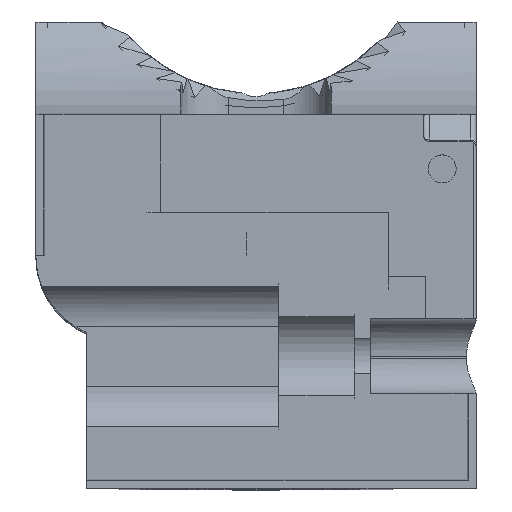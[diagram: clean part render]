
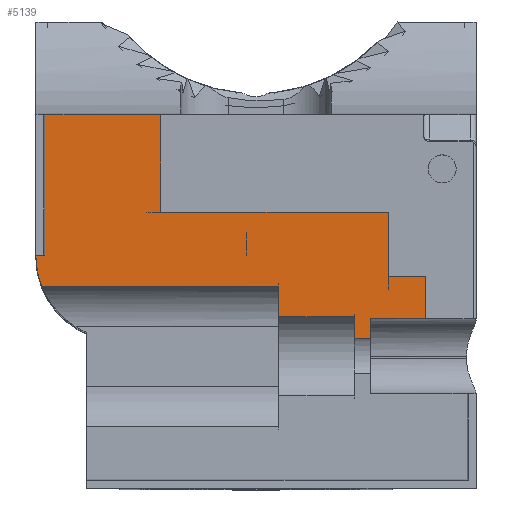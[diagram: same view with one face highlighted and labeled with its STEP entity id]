
A CAD part, top view. The second image highlights one B-rep face of the part: STEP entity #5139.
In plain terms, the highlighted planar face has unit normal (0, 0, 1).
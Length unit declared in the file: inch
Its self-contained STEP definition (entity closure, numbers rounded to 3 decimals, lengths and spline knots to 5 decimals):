
#11 = DIRECTION ( 'NONE',  ( 0., 0., -1. ) ) ;
#239 = LINE ( 'NONE', #12448, #16419 ) ;
#343 = CARTESIAN_POINT ( 'NONE',  ( 0.41447, 1.005, 0.26517 ) ) ;
#524 = VERTEX_POINT ( 'NONE', #3653 ) ;
#596 = EDGE_CURVE ( 'NONE', #15322, #9496, #13801, .T. ) ;
#885 = EDGE_CURVE ( 'NONE', #14929, #524, #7992, .T. ) ;
#1138 = LINE ( 'NONE', #10330, #13542 ) ;
#1209 = EDGE_LOOP ( 'NONE', ( #4483, #14083, #12422, #17195, #19235, #19727, #6676, #20400, #9826, #13879, #11417, #12437, #3970, #17116, #18601, #19387 ) ) ;
#1357 = VECTOR ( 'NONE', #20922, 39.37008 ) ;
#1849 = EDGE_CURVE ( 'NONE', #14929, #4978, #15786, .T. ) ;
#2146 = DIRECTION ( 'NONE',  ( -1., 0., 0. ) ) ;
#2294 = VECTOR ( 'NONE', #8218, 39.37008 ) ;
#2532 = LINE ( 'NONE', #8568, #14914 ) ;
#2558 = CARTESIAN_POINT ( 'NONE',  ( -0.03355, 0.86284, 0.26517 ) ) ;
#2764 = CARTESIAN_POINT ( 'NONE',  ( 0.41447, 1.005, 0.26517 ) ) ;
#2931 = CARTESIAN_POINT ( 'NONE',  ( 0.73097, 0.7935, 0.26517 ) ) ;
#2979 = AXIS2_PLACEMENT_3D ( 'NONE', #6484, #11, #11354 ) ;
#3005 = CARTESIAN_POINT ( 'NONE',  ( 1.05697, 0.58511, 0.26517 ) ) ;
#3012 = CARTESIAN_POINT ( 'NONE',  ( 0.80697, 1.0895, 0.26517 ) ) ;
#3136 = PLANE ( 'NONE',  #2979 ) ;
#3427 = CARTESIAN_POINT ( 'NONE',  ( 1.05697, 0.65914, 0.26517 ) ) ;
#3461 = VERTEX_POINT ( 'NONE', #8194 ) ;
#3519 = CARTESIAN_POINT ( 'NONE',  ( 1.29347, 0.6525, 0.26517 ) ) ;
#3653 = CARTESIAN_POINT ( 'NONE',  ( 0.41447, 1.33016, 0.26517 ) ) ;
#3688 = VERTEX_POINT ( 'NONE', #3519 ) ;
#3970 = ORIENTED_EDGE ( 'NONE', *, *, #596, .T. ) ;
#4374 = DIRECTION ( 'NONE',  ( 0., 1., 0. ) ) ;
#4483 = ORIENTED_EDGE ( 'NONE', *, *, #1849, .T. ) ;
#4570 = VERTEX_POINT ( 'NONE', #18582 ) ;
#4710 = LINE ( 'NONE', #2931, #11773 ) ;
#4714 = CARTESIAN_POINT ( 'NONE',  ( 0.03, 0.86284, 0.26517 ) ) ;
#4978 = VERTEX_POINT ( 'NONE', #4714 ) ;
#5139 = ADVANCED_FACE ( 'NONE', ( #8141 ), #3136, .F. ) ;
#5187 = CIRCLE ( 'NONE', #5200, 0.27784 ) ;
#5200 = AXIS2_PLACEMENT_3D ( 'NONE', #16273, #6629, #17899 ) ;
#5302 = CARTESIAN_POINT ( 'NONE',  ( 1.17047, 1.005, 0.26517 ) ) ;
#5389 = VERTEX_POINT ( 'NONE', #3427 ) ;
#5598 = VECTOR ( 'NONE', #17333, 39.37008 ) ;
#6075 = EDGE_CURVE ( 'NONE', #10537, #3461, #14701, .T. ) ;
#6139 = EDGE_CURVE ( 'NONE', #6248, #524, #9895, .T. ) ;
#6248 = VERTEX_POINT ( 'NONE', #343 ) ;
#6427 = CARTESIAN_POINT ( 'NONE',  ( 1.17047, 0.7935, 0.26517 ) ) ;
#6484 = CARTESIAN_POINT ( 'NONE',  ( -0.03355, 0.09, 0.26517 ) ) ;
#6497 = DIRECTION ( 'NONE',  ( -1., 0., 0. ) ) ;
#6609 = CARTESIAN_POINT ( 'NONE',  ( 0.80697, 0.76039, 0.26517 ) ) ;
#6629 = DIRECTION ( 'NONE',  ( 0., 0., 1. ) ) ;
#6676 = ORIENTED_EDGE ( 'NONE', *, *, #11280, .F. ) ;
#6910 = DIRECTION ( 'NONE',  ( 0., 1., 0. ) ) ;
#7098 = DIRECTION ( 'NONE',  ( -1., 0., 0. ) ) ;
#7710 = VECTOR ( 'NONE', #15720, 39.37008 ) ;
#7992 = LINE ( 'NONE', #15144, #20320 ) ;
#8141 = FACE_OUTER_BOUND ( 'NONE', #1209, .T. ) ;
#8194 = CARTESIAN_POINT ( 'NONE',  ( 0.01958, 0.76039, 0.26517 ) ) ;
#8218 = DIRECTION ( 'NONE',  ( -1., 0., 0. ) ) ;
#8321 = EDGE_CURVE ( 'NONE', #10902, #3688, #239, .T. ) ;
#8479 = VECTOR ( 'NONE', #6910, 39.37008 ) ;
#8568 = CARTESIAN_POINT ( 'NONE',  ( 1.46194, 0.6525, 0.26517 ) ) ;
#8717 = VECTOR ( 'NONE', #9055, 39.37008 ) ;
#9055 = DIRECTION ( 'NONE',  ( -1., 0., 0. ) ) ;
#9168 = DIRECTION ( 'NONE',  ( 0., -1., 0. ) ) ;
#9496 = VERTEX_POINT ( 'NONE', #15086 ) ;
#9735 = VECTOR ( 'NONE', #19088, 39.37008 ) ;
#9826 = ORIENTED_EDGE ( 'NONE', *, *, #17679, .T. ) ;
#9895 = LINE ( 'NONE', #2764, #5598 ) ;
#9969 = LINE ( 'NONE', #11279, #1357 ) ;
#10330 = CARTESIAN_POINT ( 'NONE',  ( 0.80697, 0.65914, 0.26517 ) ) ;
#10537 = VERTEX_POINT ( 'NONE', #13240 ) ;
#10554 = VERTEX_POINT ( 'NONE', #11617 ) ;
#10902 = VERTEX_POINT ( 'NONE', #13305 ) ;
#11279 = CARTESIAN_POINT ( 'NONE',  ( 0.80697, 0.58511, 0.26517 ) ) ;
#11280 = EDGE_CURVE ( 'NONE', #16374, #5389, #20043, .T. ) ;
#11354 = DIRECTION ( 'NONE',  ( -1., 0., 0. ) ) ;
#11417 = ORIENTED_EDGE ( 'NONE', *, *, #8321, .F. ) ;
#11617 = CARTESIAN_POINT ( 'NONE',  ( 0.80697, 0.65914, 0.26517 ) ) ;
#11773 = VECTOR ( 'NONE', #14239, 39.37008 ) ;
#11917 = DIRECTION ( 'NONE',  ( 1., 0., 0. ) ) ;
#12010 = VECTOR ( 'NONE', #4374, 39.37008 ) ;
#12422 = ORIENTED_EDGE ( 'NONE', *, *, #13907, .T. ) ;
#12437 = ORIENTED_EDGE ( 'NONE', *, *, #17137, .T. ) ;
#12448 = CARTESIAN_POINT ( 'NONE',  ( 1.29347, 1.0895, 0.26517 ) ) ;
#13240 = CARTESIAN_POINT ( 'NONE',  ( 0.80697, 0.76039, 0.26517 ) ) ;
#13305 = CARTESIAN_POINT ( 'NONE',  ( 1.29347, 0.7935, 0.26517 ) ) ;
#13428 = VERTEX_POINT ( 'NONE', #18507 ) ;
#13542 = VECTOR ( 'NONE', #7098, 39.37008 ) ;
#13766 = EDGE_CURVE ( 'NONE', #13428, #16374, #9969, .T. ) ;
#13801 = LINE ( 'NONE', #5302, #8479 ) ;
#13879 = ORIENTED_EDGE ( 'NONE', *, *, #18606, .F. ) ;
#13907 = EDGE_CURVE ( 'NONE', #20911, #3461, #5187, .T. ) ;
#14026 = LINE ( 'NONE', #3012, #9735 ) ;
#14041 = CARTESIAN_POINT ( 'NONE',  ( 1.05697, 0.5275, 0.26517 ) ) ;
#14083 = ORIENTED_EDGE ( 'NONE', *, *, #16069, .T. ) ;
#14239 = DIRECTION ( 'NONE',  ( -1., 0., 0. ) ) ;
#14616 = EDGE_CURVE ( 'NONE', #9496, #6248, #19795, .T. ) ;
#14701 = LINE ( 'NONE', #6609, #2294 ) ;
#14914 = VECTOR ( 'NONE', #2146, 39.37008 ) ;
#14929 = VERTEX_POINT ( 'NONE', #15853 ) ;
#14951 = EDGE_CURVE ( 'NONE', #10537, #10554, #14026, .T. ) ;
#15086 = CARTESIAN_POINT ( 'NONE',  ( 1.17047, 1.005, 0.26517 ) ) ;
#15144 = CARTESIAN_POINT ( 'NONE',  ( 1.46311, 1.33016, 0.26517 ) ) ;
#15322 = VERTEX_POINT ( 'NONE', #6427 ) ;
#15539 = VECTOR ( 'NONE', #6497, 39.37008 ) ;
#15685 = VECTOR ( 'NONE', #16545, 39.37008 ) ;
#15720 = DIRECTION ( 'NONE',  ( 0., -1., 0. ) ) ;
#15786 = LINE ( 'NONE', #15789, #7710 ) ;
#15789 = CARTESIAN_POINT ( 'NONE',  ( 0.03, 0.09, 0.26517 ) ) ;
#15853 = CARTESIAN_POINT ( 'NONE',  ( 0.03, 1.33016, 0.26517 ) ) ;
#15881 = EDGE_CURVE ( 'NONE', #5389, #10554, #1138, .T. ) ;
#16069 = EDGE_CURVE ( 'NONE', #4978, #20911, #16797, .T. ) ;
#16273 = CARTESIAN_POINT ( 'NONE',  ( 0.27784, 0.86284, 0.26517 ) ) ;
#16374 = VERTEX_POINT ( 'NONE', #3005 ) ;
#16419 = VECTOR ( 'NONE', #9168, 39.37008 ) ;
#16545 = DIRECTION ( 'NONE',  ( 0., 1., 0. ) ) ;
#16797 = LINE ( 'NONE', #2558, #8717 ) ;
#17116 = ORIENTED_EDGE ( 'NONE', *, *, #14616, .T. ) ;
#17137 = EDGE_CURVE ( 'NONE', #10902, #15322, #4710, .T. ) ;
#17195 = ORIENTED_EDGE ( 'NONE', *, *, #6075, .F. ) ;
#17333 = DIRECTION ( 'NONE',  ( 0., 1., 0. ) ) ;
#17679 = EDGE_CURVE ( 'NONE', #13428, #4570, #19945, .T. ) ;
#17692 = CARTESIAN_POINT ( 'NONE',  ( 0.73097, 1.005, 0.26517 ) ) ;
#17899 = DIRECTION ( 'NONE',  ( -1., 0., 0. ) ) ;
#18107 = CARTESIAN_POINT ( 'NONE',  ( 1.11047, 1.0895, 0.26517 ) ) ;
#18507 = CARTESIAN_POINT ( 'NONE',  ( 1.11047, 0.58511, 0.26517 ) ) ;
#18582 = CARTESIAN_POINT ( 'NONE',  ( 1.11047, 0.6525, 0.26517 ) ) ;
#18601 = ORIENTED_EDGE ( 'NONE', *, *, #6139, .T. ) ;
#18606 = EDGE_CURVE ( 'NONE', #3688, #4570, #2532, .T. ) ;
#19088 = DIRECTION ( 'NONE',  ( 0., -1., 0. ) ) ;
#19235 = ORIENTED_EDGE ( 'NONE', *, *, #14951, .T. ) ;
#19387 = ORIENTED_EDGE ( 'NONE', *, *, #885, .F. ) ;
#19416 = CARTESIAN_POINT ( 'NONE',  ( 0., 0.86284, 0.26517 ) ) ;
#19727 = ORIENTED_EDGE ( 'NONE', *, *, #15881, .F. ) ;
#19795 = LINE ( 'NONE', #17692, #15539 ) ;
#19945 = LINE ( 'NONE', #18107, #15685 ) ;
#20043 = LINE ( 'NONE', #14041, #12010 ) ;
#20320 = VECTOR ( 'NONE', #11917, 39.37008 ) ;
#20400 = ORIENTED_EDGE ( 'NONE', *, *, #13766, .F. ) ;
#20911 = VERTEX_POINT ( 'NONE', #19416 ) ;
#20922 = DIRECTION ( 'NONE',  ( -1., 0., 0. ) ) ;
